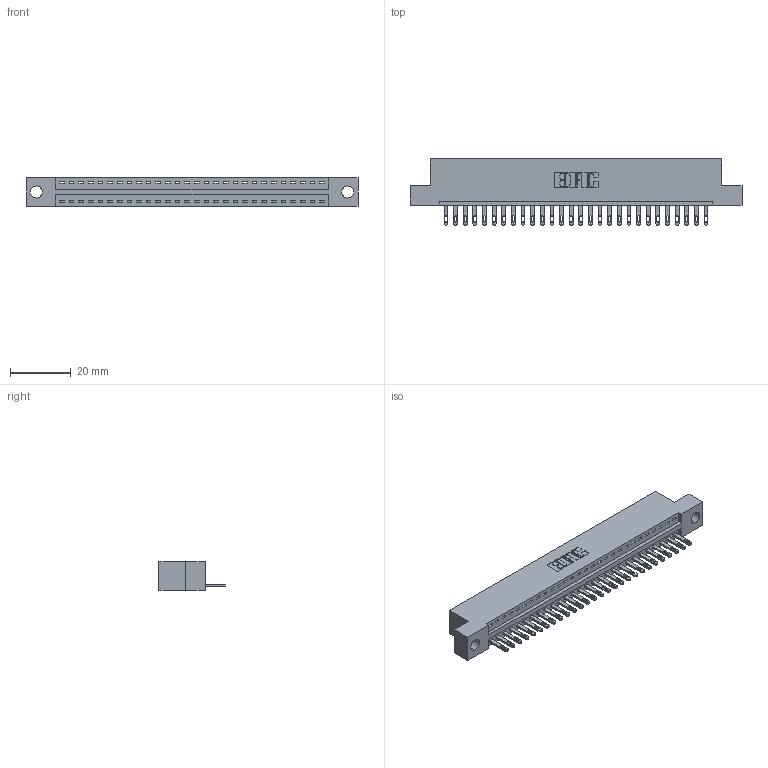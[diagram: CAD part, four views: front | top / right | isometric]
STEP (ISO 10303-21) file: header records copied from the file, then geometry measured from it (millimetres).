
FILE_DESCRIPTION (( 'STEP AP203' ), '1' );
FILE_NAME ('896-028-500-104.STEP', '2021-07-27T18:16:05', ( '' ), ( '' ), 'SwSTEP 2.0', 'SolidWorks 2020', '' );
FILE_SCHEMA (( 'CONFIG_CONTROL_DESIGN' ));
Length unit declared in the file: inch
Products named in the file (3): 345-292-001_345-293-100; 846 Part_Flush Mounting Lugs - 0.156 Dia-TH; 896-028-500-104
Assembly tree (29 placements, depth 2):
  896-028-500-104
    846 Part_Flush Mounting Lugs - 0.156 Dia-TH
    345-292-001_345-293-100  x28
Bounding box: 109.47 x 21.84 x 9.4 mm (x, y, z)
Volume: 10312.1 mm3; surface area: 12607.9 mm2
Topology: 29 solids, 29 shells, 1634 faces, 5033 edges, 3354 vertices
Faces by surface type: plane 1028, cylinder 606
Entity records: 19195 total; most frequent: CARTESIAN_POINT 3300, ORIENTED_EDGE 3262, DIRECTION 2931, EDGE_CURVE 1631, VECTOR 1383, LINE 1383, VERTEX_POINT 1086, AXIS2_PLACEMENT_3D 774
